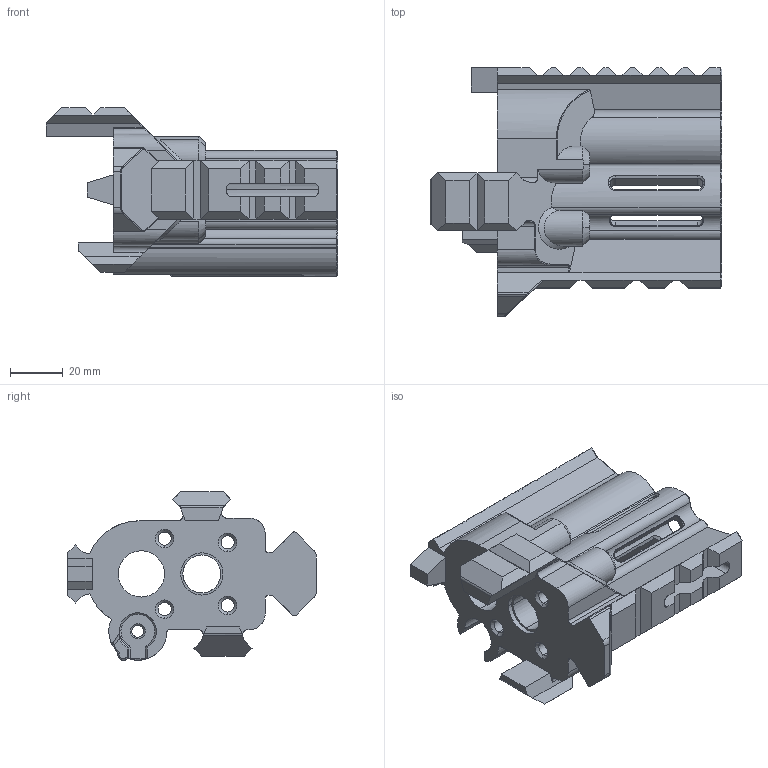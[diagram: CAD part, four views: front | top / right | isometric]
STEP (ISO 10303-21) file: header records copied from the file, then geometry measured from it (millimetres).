
FILE_DESCRIPTION (( 'STEP AP203' ), '1' );
FILE_NAME ('MOD9_V3_Barrel_Retainer.STEP', '2020-12-23T22:04:22', ( '' ), ( '' ), 'SwSTEP 2.0', 'SolidWorks 2019', '' );
FILE_SCHEMA (( 'CONFIG_CONTROL_DESIGN' ));
Length unit declared in the file: millimetre
Products named in the file (1): MOD9_V3_Barrel_Retainer
Bounding box: 110.59 x 94.2 x 63.85 mm (x, y, z)
Volume: 147287.8 mm3; surface area: 47553.4 mm2
Topology: 1 solids, 1 shells, 472 faces, 1221 edges, 746 vertices
Faces by surface type: plane 184, cylinder 129, bspline 88, cone 71
Entity records: 19538 total; most frequent: CARTESIAN_POINT 8799, ORIENTED_EDGE 2434, DIRECTION 1899, EDGE_CURVE 1217, VERTEX_POINT 746, LINE 665, VECTOR 665, AXIS2_PLACEMENT_3D 617
